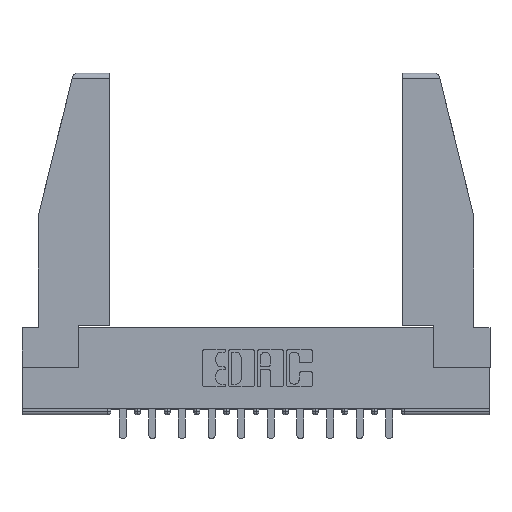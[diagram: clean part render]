
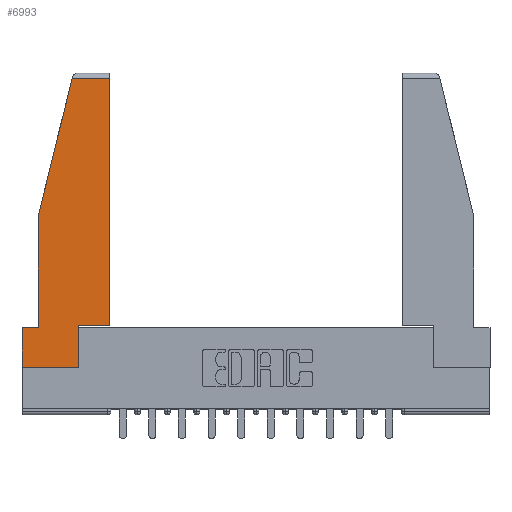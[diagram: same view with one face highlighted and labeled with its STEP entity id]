
A CAD part, top view. The second image highlights one B-rep face of the part: STEP entity #6993.
In plain terms, the highlighted planar face has unit normal (0, 0, 1).
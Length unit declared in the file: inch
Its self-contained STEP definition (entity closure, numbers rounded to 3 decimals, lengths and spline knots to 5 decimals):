
#17 = VECTOR ( 'NONE', #15445, 39.37008 ) ;
#669 = DIRECTION ( 'NONE',  ( -0.239, -0.971, 0. ) ) ;
#1007 = EDGE_CURVE ( 'NONE', #4930, #3639, #6506, .T. ) ;
#1422 = LINE ( 'NONE', #11033, #11424 ) ;
#1454 = DIRECTION ( 'NONE',  ( 1., 0., 0. ) ) ;
#1537 = DIRECTION ( 'NONE',  ( 0., 0., 1. ) ) ;
#1606 = EDGE_CURVE ( 'NONE', #3639, #6595, #15138, .T. ) ;
#1695 = EDGE_CURVE ( 'NONE', #8856, #6300, #12480, .T. ) ;
#1979 = ORIENTED_EDGE ( 'NONE', *, *, #9413, .T. ) ;
#2018 = CARTESIAN_POINT ( 'NONE',  ( 0.461, 0.223, 0. ) ) ;
#2424 = VERTEX_POINT ( 'NONE', #4612 ) ;
#2477 = CARTESIAN_POINT ( 'NONE',  ( 0., 0.21, 0. ) ) ;
#2520 = CARTESIAN_POINT ( 'NONE',  ( 0.086, 0.8, 0. ) ) ;
#2560 = ORIENTED_EDGE ( 'NONE', *, *, #1695, .T. ) ;
#2575 = VECTOR ( 'NONE', #15839, 39.37008 ) ;
#2601 = EDGE_CURVE ( 'NONE', #6300, #2424, #14146, .T. ) ;
#2971 = CARTESIAN_POINT ( 'NONE',  ( 0., 0.21, 0. ) ) ;
#3260 = ORIENTED_EDGE ( 'NONE', *, *, #2601, .T. ) ;
#3555 = CARTESIAN_POINT ( 'NONE',  ( 0.2636, 1.52, 0. ) ) ;
#3639 = VERTEX_POINT ( 'NONE', #3870 ) ;
#3675 = LINE ( 'NONE', #2971, #13102 ) ;
#3870 = CARTESIAN_POINT ( 'NONE',  ( 0.297, 0.223, 0. ) ) ;
#4123 = VERTEX_POINT ( 'NONE', #13553 ) ;
#4461 = EDGE_CURVE ( 'NONE', #14280, #4930, #1422, .T. ) ;
#4612 = CARTESIAN_POINT ( 'NONE',  ( 0.086, 0.21, 0. ) ) ;
#4930 = VERTEX_POINT ( 'NONE', #13881 ) ;
#5332 = CARTESIAN_POINT ( 'NONE',  ( 0., 0., 0. ) ) ;
#5404 = CARTESIAN_POINT ( 'NONE',  ( 0.086, 0.8, 0. ) ) ;
#5957 = CARTESIAN_POINT ( 'NONE',  ( 0., 0.21, 0. ) ) ;
#6002 = DIRECTION ( 'NONE',  ( -1., 0., 0. ) ) ;
#6162 = DIRECTION ( 'NONE',  ( 1., 0., 0. ) ) ;
#6300 = VERTEX_POINT ( 'NONE', #2520 ) ;
#6387 = LINE ( 'NONE', #2477, #7940 ) ;
#6506 = LINE ( 'NONE', #14258, #17 ) ;
#6595 = VERTEX_POINT ( 'NONE', #2018 ) ;
#6787 = ORIENTED_EDGE ( 'NONE', *, *, #8709, .T. ) ;
#6949 = AXIS2_PLACEMENT_3D ( 'NONE', #15029, #1537, #12594 ) ;
#6993 = ADVANCED_FACE ( 'NONE', ( #9548 ), #9015, .T. ) ;
#7239 = VECTOR ( 'NONE', #12784, 39.37008 ) ;
#7367 = LINE ( 'NONE', #12552, #9471 ) ;
#7716 = ORIENTED_EDGE ( 'NONE', *, *, #4461, .T. ) ;
#7873 = EDGE_LOOP ( 'NONE', ( #1979, #6787, #2560, #3260, #7969, #8693, #7716, #8481, #8772 ) ) ;
#7940 = VECTOR ( 'NONE', #6002, 39.37008 ) ;
#7969 = ORIENTED_EDGE ( 'NONE', *, *, #8786, .T. ) ;
#8481 = ORIENTED_EDGE ( 'NONE', *, *, #1007, .T. ) ;
#8693 = ORIENTED_EDGE ( 'NONE', *, *, #15468, .T. ) ;
#8709 = EDGE_CURVE ( 'NONE', #4123, #8856, #11239, .T. ) ;
#8772 = ORIENTED_EDGE ( 'NONE', *, *, #1606, .T. ) ;
#8786 = EDGE_CURVE ( 'NONE', #2424, #15844, #6387, .T. ) ;
#8856 = VERTEX_POINT ( 'NONE', #3555 ) ;
#9015 = PLANE ( 'NONE',  #6949 ) ;
#9168 = VECTOR ( 'NONE', #669, 39.37008 ) ;
#9413 = EDGE_CURVE ( 'NONE', #6595, #4123, #7367, .T. ) ;
#9471 = VECTOR ( 'NONE', #14930, 39.37008 ) ;
#9548 = FACE_OUTER_BOUND ( 'NONE', #7873, .T. ) ;
#9656 = CARTESIAN_POINT ( 'NONE',  ( 0., 1.52, 0. ) ) ;
#11033 = CARTESIAN_POINT ( 'NONE',  ( 0., 0., 0. ) ) ;
#11239 = LINE ( 'NONE', #9656, #2575 ) ;
#11328 = VECTOR ( 'NONE', #1454, 39.37008 ) ;
#11424 = VECTOR ( 'NONE', #6162, 39.37008 ) ;
#12480 = LINE ( 'NONE', #15355, #9168 ) ;
#12552 = CARTESIAN_POINT ( 'NONE',  ( 0.461, 0.223, 0. ) ) ;
#12594 = DIRECTION ( 'NONE',  ( 1., 0., 0. ) ) ;
#12687 = CARTESIAN_POINT ( 'NONE',  ( 0.297, 0.223, 0. ) ) ;
#12784 = DIRECTION ( 'NONE',  ( 0., -1., 0. ) ) ;
#13102 = VECTOR ( 'NONE', #14363, 39.37008 ) ;
#13553 = CARTESIAN_POINT ( 'NONE',  ( 0.461, 1.52, 0. ) ) ;
#13881 = CARTESIAN_POINT ( 'NONE',  ( 0.297, 0., 0. ) ) ;
#14146 = LINE ( 'NONE', #5404, #7239 ) ;
#14258 = CARTESIAN_POINT ( 'NONE',  ( 0.297, 0., 0. ) ) ;
#14280 = VERTEX_POINT ( 'NONE', #5332 ) ;
#14363 = DIRECTION ( 'NONE',  ( 0., -1., 0. ) ) ;
#14930 = DIRECTION ( 'NONE',  ( 0., 1., 0. ) ) ;
#15029 = CARTESIAN_POINT ( 'NONE',  ( 0., 0., 0. ) ) ;
#15138 = LINE ( 'NONE', #12687, #11328 ) ;
#15355 = CARTESIAN_POINT ( 'NONE',  ( 0.271, 1.55, 0. ) ) ;
#15445 = DIRECTION ( 'NONE',  ( 0., 1., 0. ) ) ;
#15468 = EDGE_CURVE ( 'NONE', #15844, #14280, #3675, .T. ) ;
#15839 = DIRECTION ( 'NONE',  ( -1., 0., 0. ) ) ;
#15844 = VERTEX_POINT ( 'NONE', #5957 ) ;
